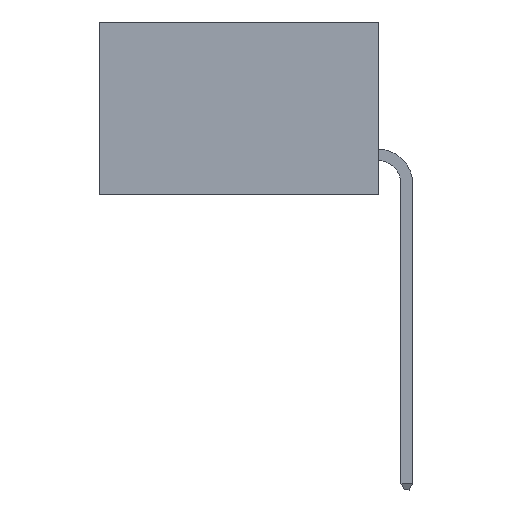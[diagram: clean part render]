
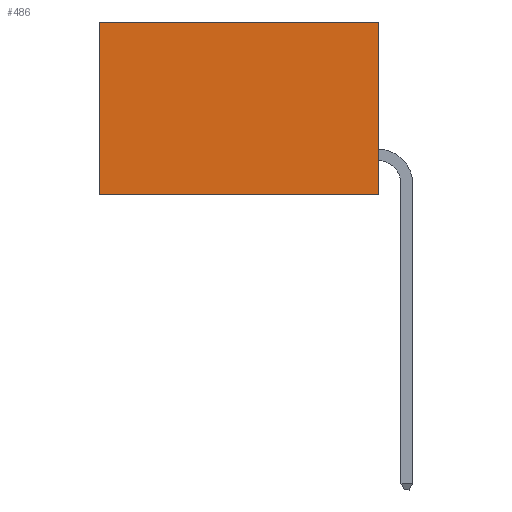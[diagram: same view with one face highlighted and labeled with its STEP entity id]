
A CAD part, left-side view. The second image highlights one B-rep face of the part: STEP entity #486.
In plain terms, the highlighted planar face has unit normal (-1, 0, 0).
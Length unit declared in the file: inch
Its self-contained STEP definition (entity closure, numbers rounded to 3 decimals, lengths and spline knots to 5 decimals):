
#486 = ADVANCED_FACE ( 'NONE', ( #7616 ), #9037, .F. ) ;
#2702 = CARTESIAN_POINT ( 'NONE',  ( 0.298, 0.6, 0. ) ) ;
#3166 = VERTEX_POINT ( 'NONE', #20182 ) ;
#4583 = AXIS2_PLACEMENT_3D ( 'NONE', #9784, #7611, #7247 ) ;
#5640 = VERTEX_POINT ( 'NONE', #21707 ) ;
#5684 = LINE ( 'NONE', #20237, #17339 ) ;
#6129 = EDGE_CURVE ( 'NONE', #3166, #7846, #28146, .T. ) ;
#6758 = DIRECTION ( 'NONE',  ( 0., 0., -1. ) ) ;
#7247 = DIRECTION ( 'NONE',  ( 0., 0., -1. ) ) ;
#7611 = DIRECTION ( 'NONE',  ( 1., 0., 0. ) ) ;
#7616 = FACE_OUTER_BOUND ( 'NONE', #15928, .T. ) ;
#7846 = VERTEX_POINT ( 'NONE', #9100 ) ;
#8342 = VERTEX_POINT ( 'NONE', #26787 ) ;
#8680 = DIRECTION ( 'NONE',  ( 0., 0., -1. ) ) ;
#9037 = PLANE ( 'NONE',  #4583 ) ;
#9100 = CARTESIAN_POINT ( 'NONE',  ( 0.298, 0.6, -0.37 ) ) ;
#9784 = CARTESIAN_POINT ( 'NONE',  ( 0.298, 0., 0. ) ) ;
#10910 = LINE ( 'NONE', #18163, #22470 ) ;
#11741 = ORIENTED_EDGE ( 'NONE', *, *, #6129, .T. ) ;
#11988 = DIRECTION ( 'NONE',  ( 0., 1., 0. ) ) ;
#13616 = DIRECTION ( 'NONE',  ( 0., 1., 0. ) ) ;
#14291 = EDGE_CURVE ( 'NONE', #5640, #3166, #23119, .T. ) ;
#15928 = EDGE_LOOP ( 'NONE', ( #11741, #20532, #28513, #29701 ) ) ;
#17022 = VECTOR ( 'NONE', #11988, 39.37008 ) ;
#17339 = VECTOR ( 'NONE', #8680, 39.37008 ) ;
#18163 = CARTESIAN_POINT ( 'NONE',  ( 0.298, 0., -0.37 ) ) ;
#20182 = CARTESIAN_POINT ( 'NONE',  ( 0.298, 0.6, 0. ) ) ;
#20237 = CARTESIAN_POINT ( 'NONE',  ( 0.298, 0., 0. ) ) ;
#20532 = ORIENTED_EDGE ( 'NONE', *, *, #28315, .F. ) ;
#21408 = VECTOR ( 'NONE', #6758, 39.37008 ) ;
#21707 = CARTESIAN_POINT ( 'NONE',  ( 0.298, 0., 0. ) ) ;
#22470 = VECTOR ( 'NONE', #13616, 39.37008 ) ;
#23119 = LINE ( 'NONE', #28000, #17022 ) ;
#25863 = EDGE_CURVE ( 'NONE', #5640, #8342, #5684, .T. ) ;
#26787 = CARTESIAN_POINT ( 'NONE',  ( 0.298, 0., -0.37 ) ) ;
#28000 = CARTESIAN_POINT ( 'NONE',  ( 0.298, 0., 0. ) ) ;
#28146 = LINE ( 'NONE', #2702, #21408 ) ;
#28315 = EDGE_CURVE ( 'NONE', #8342, #7846, #10910, .T. ) ;
#28513 = ORIENTED_EDGE ( 'NONE', *, *, #25863, .F. ) ;
#29701 = ORIENTED_EDGE ( 'NONE', *, *, #14291, .T. ) ;
